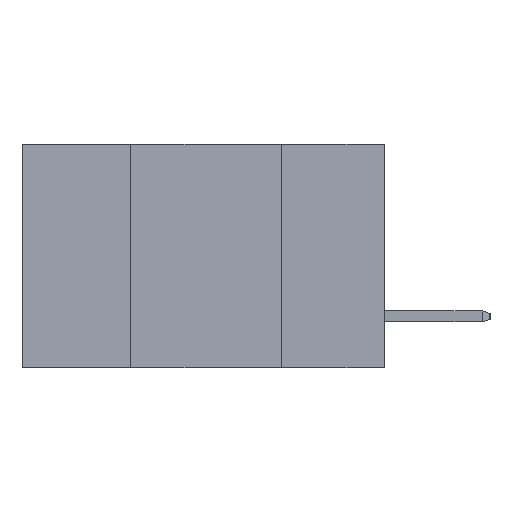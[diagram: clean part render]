
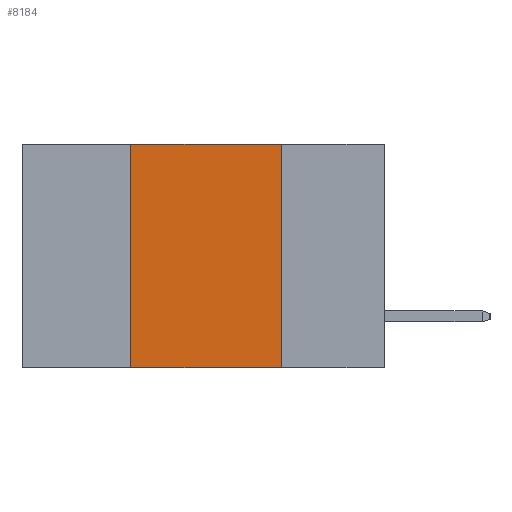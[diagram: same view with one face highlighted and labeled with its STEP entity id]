
A CAD part, left-side view. The second image highlights one B-rep face of the part: STEP entity #8184.
In plain terms, the highlighted planar face has unit normal (-1, 0, 0).
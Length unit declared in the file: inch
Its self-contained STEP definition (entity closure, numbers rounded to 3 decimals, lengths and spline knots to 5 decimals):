
#2073 = VERTEX_POINT ( 'NONE', #2302 ) ;
#2205 = VECTOR ( 'NONE', #5989, 39.37008 ) ;
#2302 = CARTESIAN_POINT ( 'NONE',  ( 0., 0.42, -0.37 ) ) ;
#2370 = ORIENTED_EDGE ( 'NONE', *, *, #17240, .T. ) ;
#2375 = EDGE_LOOP ( 'NONE', ( #5830, #9150, #8807, #2370 ) ) ;
#2957 = AXIS2_PLACEMENT_3D ( 'NONE', #7296, #15440, #7365 ) ;
#3353 = VERTEX_POINT ( 'NONE', #10524 ) ;
#3401 = VECTOR ( 'NONE', #3411, 39.37008 ) ;
#3411 = DIRECTION ( 'NONE',  ( 0., -1., 0. ) ) ;
#3839 = LINE ( 'NONE', #4846, #3401 ) ;
#4846 = CARTESIAN_POINT ( 'NONE',  ( 0., 0.6, 0. ) ) ;
#5830 = ORIENTED_EDGE ( 'NONE', *, *, #16037, .F. ) ;
#5912 = PLANE ( 'NONE',  #2957 ) ;
#5965 = VERTEX_POINT ( 'NONE', #15905 ) ;
#5989 = DIRECTION ( 'NONE',  ( 0., -1., 0. ) ) ;
#6148 = EDGE_CURVE ( 'NONE', #2073, #3353, #12371, .T. ) ;
#6998 = LINE ( 'NONE', #8087, #17391 ) ;
#7296 = CARTESIAN_POINT ( 'NONE',  ( 0., 0.6, 0. ) ) ;
#7365 = DIRECTION ( 'NONE',  ( 0., 0., -1. ) ) ;
#7439 = CARTESIAN_POINT ( 'NONE',  ( 0., 0.6, -0.37 ) ) ;
#8087 = CARTESIAN_POINT ( 'NONE',  ( 0., 0.17, 0. ) ) ;
#8184 = ADVANCED_FACE ( 'NONE', ( #15977 ), #5912, .F. ) ;
#8807 = ORIENTED_EDGE ( 'NONE', *, *, #6148, .F. ) ;
#9150 = ORIENTED_EDGE ( 'NONE', *, *, #11101, .F. ) ;
#9544 = DIRECTION ( 'NONE',  ( 0., 0., -1. ) ) ;
#9915 = VERTEX_POINT ( 'NONE', #10422 ) ;
#10422 = CARTESIAN_POINT ( 'NONE',  ( 0., 0.17, -0.37 ) ) ;
#10524 = CARTESIAN_POINT ( 'NONE',  ( 0., 0.42, 0. ) ) ;
#11101 = EDGE_CURVE ( 'NONE', #3353, #5965, #3839, .T. ) ;
#11949 = VECTOR ( 'NONE', #16042, 39.37008 ) ;
#12371 = LINE ( 'NONE', #13382, #11949 ) ;
#13297 = LINE ( 'NONE', #7439, #2205 ) ;
#13382 = CARTESIAN_POINT ( 'NONE',  ( 0., 0.42, 0. ) ) ;
#15440 = DIRECTION ( 'NONE',  ( 1., 0., 0. ) ) ;
#15905 = CARTESIAN_POINT ( 'NONE',  ( 0., 0.17, 0. ) ) ;
#15977 = FACE_OUTER_BOUND ( 'NONE', #2375, .T. ) ;
#16037 = EDGE_CURVE ( 'NONE', #5965, #9915, #6998, .T. ) ;
#16042 = DIRECTION ( 'NONE',  ( 0., 0., 1. ) ) ;
#17240 = EDGE_CURVE ( 'NONE', #2073, #9915, #13297, .T. ) ;
#17391 = VECTOR ( 'NONE', #9544, 39.37008 ) ;
